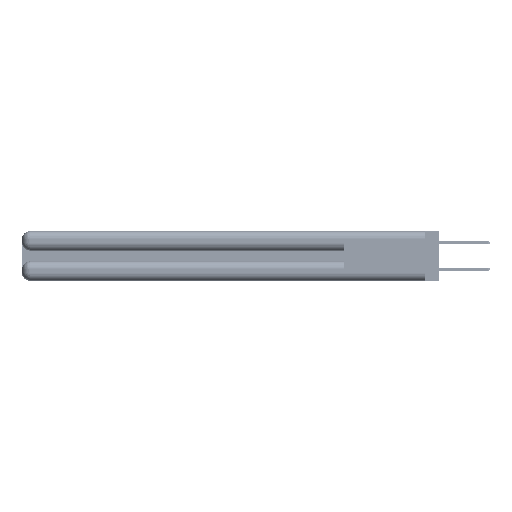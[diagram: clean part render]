
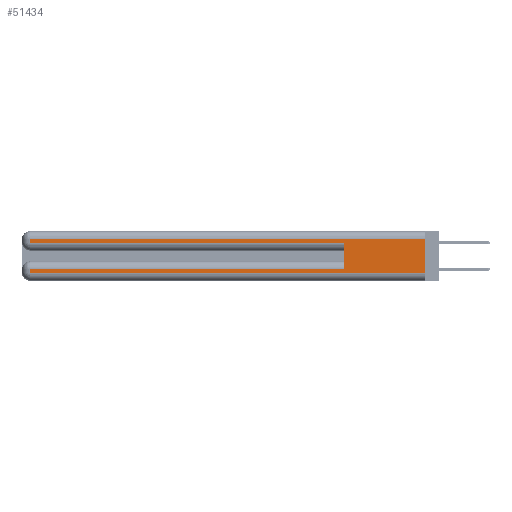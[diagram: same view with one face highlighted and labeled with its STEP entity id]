
A CAD part, left-side view. The second image highlights one B-rep face of the part: STEP entity #51434.
In plain terms, the highlighted planar face has unit normal (-1, 0, 0).
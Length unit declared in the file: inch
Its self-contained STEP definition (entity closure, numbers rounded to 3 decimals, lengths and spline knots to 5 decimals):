
#560 = LINE ( 'NONE', #26777, #30957 ) ;
#944 = CARTESIAN_POINT ( 'NONE',  ( 0., 0., 0.37 ) ) ;
#1284 = EDGE_CURVE ( 'NONE', #49942, #46108, #12733, .T. ) ;
#2842 = CARTESIAN_POINT ( 'NONE',  ( 0., 0.6, 0.145 ) ) ;
#3410 = ORIENTED_EDGE ( 'NONE', *, *, #53723, .T. ) ;
#3869 = CARTESIAN_POINT ( 'NONE',  ( 0., 2.94, 0.37 ) ) ;
#3991 = VERTEX_POINT ( 'NONE', #33869 ) ;
#4396 = VERTEX_POINT ( 'NONE', #40790 ) ;
#4809 = CARTESIAN_POINT ( 'NONE',  ( 0., 0.6, 0.085 ) ) ;
#5206 = DIRECTION ( 'NONE',  ( 0., 0., -1. ) ) ;
#6702 = ORIENTED_EDGE ( 'NONE', *, *, #1284, .T. ) ;
#7916 = EDGE_LOOP ( 'NONE', ( #30499, #32043, #6702, #29332, #53200, #31522, #13109, #3410 ) ) ;
#9439 = DIRECTION ( 'NONE',  ( 0., -1., 0. ) ) ;
#9610 = CARTESIAN_POINT ( 'NONE',  ( 0., 0., 0.37 ) ) ;
#10248 = FACE_OUTER_BOUND ( 'NONE', #7916, .T. ) ;
#12412 = VECTOR ( 'NONE', #20217, 39.37008 ) ;
#12733 = LINE ( 'NONE', #36933, #43041 ) ;
#13109 = ORIENTED_EDGE ( 'NONE', *, *, #43413, .T. ) ;
#14229 = DIRECTION ( 'NONE',  ( 1., 0., 0. ) ) ;
#14278 = LINE ( 'NONE', #3869, #47852 ) ;
#14585 = VECTOR ( 'NONE', #17473, 39.37008 ) ;
#15628 = CARTESIAN_POINT ( 'NONE',  ( 0., 0., 0.285 ) ) ;
#16212 = AXIS2_PLACEMENT_3D ( 'NONE', #9610, #14229, #5206 ) ;
#17183 = DIRECTION ( 'NONE',  ( 0., 0., -1. ) ) ;
#17473 = DIRECTION ( 'NONE',  ( 0., 1., 0. ) ) ;
#18292 = PLANE ( 'NONE',  #16212 ) ;
#18496 = VECTOR ( 'NONE', #39365, 39.37008 ) ;
#18943 = EDGE_CURVE ( 'NONE', #4396, #26076, #48497, .T. ) ;
#19185 = LINE ( 'NONE', #22066, #14585 ) ;
#19530 = CARTESIAN_POINT ( 'NONE',  ( 0., 2.94, 0.085 ) ) ;
#20217 = DIRECTION ( 'NONE',  ( 0., 0., 1. ) ) ;
#22066 = CARTESIAN_POINT ( 'NONE',  ( 0., 0., 0.085 ) ) ;
#25188 = CARTESIAN_POINT ( 'NONE',  ( 0., 0., 0.06 ) ) ;
#26076 = VERTEX_POINT ( 'NONE', #25188 ) ;
#26147 = VECTOR ( 'NONE', #34693, 39.37008 ) ;
#26777 = CARTESIAN_POINT ( 'NONE',  ( 0., 0., 0.06 ) ) ;
#27974 = DIRECTION ( 'NONE',  ( 0., 0., -1. ) ) ;
#29332 = ORIENTED_EDGE ( 'NONE', *, *, #31321, .T. ) ;
#30499 = ORIENTED_EDGE ( 'NONE', *, *, #18943, .F. ) ;
#30957 = VECTOR ( 'NONE', #9439, 39.37008 ) ;
#31321 = EDGE_CURVE ( 'NONE', #46108, #3991, #45586, .T. ) ;
#31492 = EDGE_CURVE ( 'NONE', #45847, #43867, #19185, .T. ) ;
#31522 = ORIENTED_EDGE ( 'NONE', *, *, #31492, .T. ) ;
#32043 = ORIENTED_EDGE ( 'NONE', *, *, #41275, .T. ) ;
#33850 = DIRECTION ( 'NONE',  ( 0., -1., 0. ) ) ;
#33869 = CARTESIAN_POINT ( 'NONE',  ( 0., 0.6, 0.285 ) ) ;
#34693 = DIRECTION ( 'NONE',  ( 0., 0., -1. ) ) ;
#35130 = CARTESIAN_POINT ( 'NONE',  ( 0., 0., 0.31 ) ) ;
#36933 = CARTESIAN_POINT ( 'NONE',  ( 0., 2.94, 0.37 ) ) ;
#36973 = CARTESIAN_POINT ( 'NONE',  ( 0., 2.94, 0.285 ) ) ;
#37436 = LINE ( 'NONE', #2842, #12412 ) ;
#37527 = CARTESIAN_POINT ( 'NONE',  ( 0., 2.94, 0.31 ) ) ;
#39365 = DIRECTION ( 'NONE',  ( 0., 1., 0. ) ) ;
#40790 = CARTESIAN_POINT ( 'NONE',  ( 0., 0., 0.31 ) ) ;
#41275 = EDGE_CURVE ( 'NONE', #4396, #49942, #42177, .T. ) ;
#41588 = VECTOR ( 'NONE', #33850, 39.37008 ) ;
#42177 = LINE ( 'NONE', #35130, #18496 ) ;
#42526 = EDGE_CURVE ( 'NONE', #45847, #3991, #37436, .T. ) ;
#43041 = VECTOR ( 'NONE', #27974, 39.37008 ) ;
#43413 = EDGE_CURVE ( 'NONE', #43867, #43633, #14278, .T. ) ;
#43633 = VERTEX_POINT ( 'NONE', #51906 ) ;
#43867 = VERTEX_POINT ( 'NONE', #19530 ) ;
#45586 = LINE ( 'NONE', #15628, #41588 ) ;
#45847 = VERTEX_POINT ( 'NONE', #4809 ) ;
#46108 = VERTEX_POINT ( 'NONE', #36973 ) ;
#47852 = VECTOR ( 'NONE', #17183, 39.37008 ) ;
#48497 = LINE ( 'NONE', #944, #26147 ) ;
#49942 = VERTEX_POINT ( 'NONE', #37527 ) ;
#51434 = ADVANCED_FACE ( 'NONE', ( #10248 ), #18292, .F. ) ;
#51906 = CARTESIAN_POINT ( 'NONE',  ( 0., 2.94, 0.06 ) ) ;
#53200 = ORIENTED_EDGE ( 'NONE', *, *, #42526, .F. ) ;
#53723 = EDGE_CURVE ( 'NONE', #43633, #26076, #560, .T. ) ;
